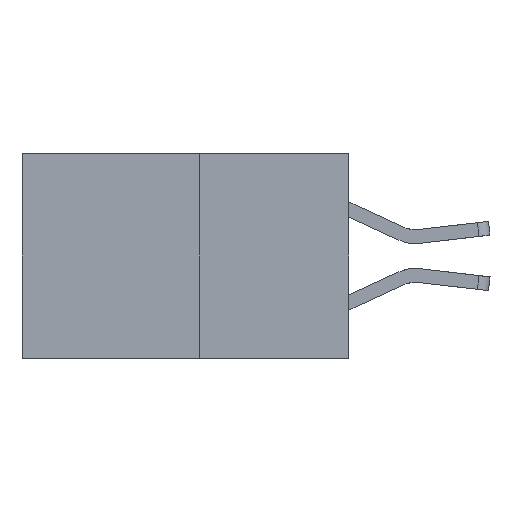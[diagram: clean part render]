
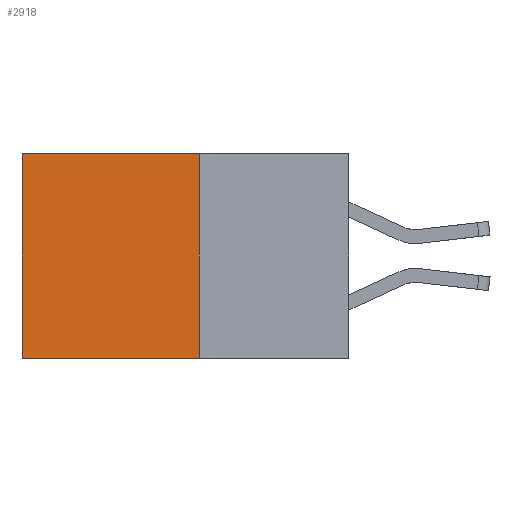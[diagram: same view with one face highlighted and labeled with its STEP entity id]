
A CAD part, left-side view. The second image highlights one B-rep face of the part: STEP entity #2918.
In plain terms, the highlighted planar face has unit normal (-1, 0, 0).
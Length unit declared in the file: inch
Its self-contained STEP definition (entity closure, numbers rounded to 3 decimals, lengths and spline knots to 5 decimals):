
#105 = CARTESIAN_POINT ( 'NONE',  ( 0.277, 0.59, -0.37 ) ) ;
#173 = LINE ( 'NONE', #7921, #6615 ) ;
#203 = DIRECTION ( 'NONE',  ( 0., 1., 0. ) ) ;
#400 = ORIENTED_EDGE ( 'NONE', *, *, #7628, .T. ) ;
#859 = CARTESIAN_POINT ( 'NONE',  ( 0.277, 0.27, 0. ) ) ;
#1452 = VERTEX_POINT ( 'NONE', #5556 ) ;
#1547 = DIRECTION ( 'NONE',  ( 0., 0., -1. ) ) ;
#2089 = CARTESIAN_POINT ( 'NONE',  ( 0.277, 0.27, 0. ) ) ;
#2177 = CARTESIAN_POINT ( 'NONE',  ( 0.277, 0.59, -0.37 ) ) ;
#2285 = EDGE_CURVE ( 'NONE', #5759, #1452, #6808, .T. ) ;
#2286 = VERTEX_POINT ( 'NONE', #105 ) ;
#2359 = FACE_OUTER_BOUND ( 'NONE', #7863, .T. ) ;
#2552 = CARTESIAN_POINT ( 'NONE',  ( 0.277, 0.27, -0.37 ) ) ;
#2827 = VERTEX_POINT ( 'NONE', #4962 ) ;
#2918 = ADVANCED_FACE ( 'NONE', ( #2359 ), #7198, .F. ) ;
#2972 = ORIENTED_EDGE ( 'NONE', *, *, #6916, .F. ) ;
#3267 = LINE ( 'NONE', #2177, #8224 ) ;
#3341 = CARTESIAN_POINT ( 'NONE',  ( 0.277, 0.27, -0.37 ) ) ;
#3598 = ORIENTED_EDGE ( 'NONE', *, *, #2285, .F. ) ;
#3729 = AXIS2_PLACEMENT_3D ( 'NONE', #3341, #7864, #3995 ) ;
#3995 = DIRECTION ( 'NONE',  ( 0., 0., -1. ) ) ;
#4055 = DIRECTION ( 'NONE',  ( 0., 1., 0. ) ) ;
#4173 = DIRECTION ( 'NONE',  ( 0., 0., -1. ) ) ;
#4194 = VECTOR ( 'NONE', #4055, 39.37008 ) ;
#4962 = CARTESIAN_POINT ( 'NONE',  ( 0.277, 0.59, 0. ) ) ;
#5314 = VECTOR ( 'NONE', #4173, 39.37008 ) ;
#5556 = CARTESIAN_POINT ( 'NONE',  ( 0.277, 0.27, -0.37 ) ) ;
#5691 = EDGE_CURVE ( 'NONE', #5759, #2827, #7832, .T. ) ;
#5759 = VERTEX_POINT ( 'NONE', #859 ) ;
#6615 = VECTOR ( 'NONE', #203, 39.37008 ) ;
#6808 = LINE ( 'NONE', #2552, #5314 ) ;
#6916 = EDGE_CURVE ( 'NONE', #1452, #2286, #173, .T. ) ;
#7198 = PLANE ( 'NONE',  #3729 ) ;
#7217 = ORIENTED_EDGE ( 'NONE', *, *, #5691, .T. ) ;
#7628 = EDGE_CURVE ( 'NONE', #2827, #2286, #3267, .T. ) ;
#7832 = LINE ( 'NONE', #2089, #4194 ) ;
#7863 = EDGE_LOOP ( 'NONE', ( #400, #2972, #3598, #7217 ) ) ;
#7864 = DIRECTION ( 'NONE',  ( 1., 0., 0. ) ) ;
#7921 = CARTESIAN_POINT ( 'NONE',  ( 0.277, 0.27, -0.37 ) ) ;
#8224 = VECTOR ( 'NONE', #1547, 39.37008 ) ;
